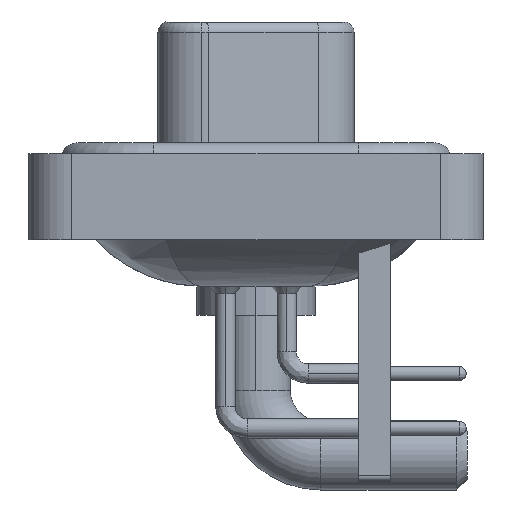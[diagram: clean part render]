
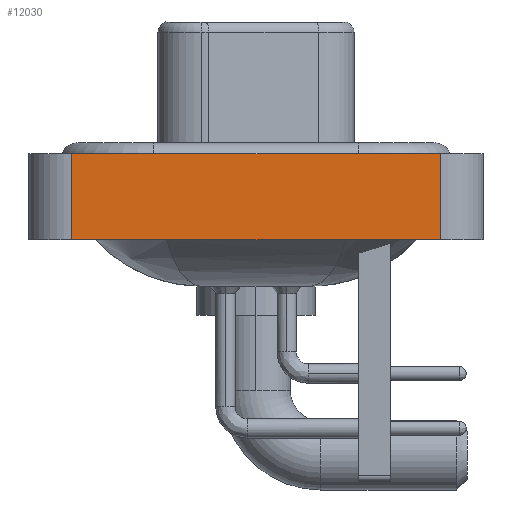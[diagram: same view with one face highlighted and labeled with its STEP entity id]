
A CAD part, left-side view. The second image highlights one B-rep face of the part: STEP entity #12030.
In plain terms, the highlighted planar face has unit normal (-1, 0, 0).
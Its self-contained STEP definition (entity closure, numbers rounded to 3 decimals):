
#790 = DIRECTION ( 'NONE',  ( 0., 0., 1. ) ) ;
#1094 = FACE_OUTER_BOUND ( 'NONE', #12705, .T. ) ;
#1133 = CARTESIAN_POINT ( 'NONE',  ( -7.3, 8.55, -3.6 ) ) ;
#2827 = CARTESIAN_POINT ( 'NONE',  ( -7.3, -8.55, 0.4 ) ) ;
#2832 = CARTESIAN_POINT ( 'NONE',  ( -7.3, -8.55, -3.6 ) ) ;
#3358 = EDGE_CURVE ( 'NONE', #23536, #13265, #13192, .T. ) ;
#3479 = CARTESIAN_POINT ( 'NONE',  ( -7.3, -8.55, -3.6 ) ) ;
#3744 = VERTEX_POINT ( 'NONE', #9728 ) ;
#3817 = VECTOR ( 'NONE', #11055, 1000. ) ;
#4490 = DIRECTION ( 'NONE',  ( 0., -1., 0. ) ) ;
#4636 = VECTOR ( 'NONE', #790, 1000. ) ;
#6869 = PLANE ( 'NONE',  #13501 ) ;
#7270 = DIRECTION ( 'NONE',  ( 0., 0., 1. ) ) ;
#9379 = EDGE_CURVE ( 'NONE', #3744, #13265, #21364, .T. ) ;
#9728 = CARTESIAN_POINT ( 'NONE',  ( -7.3, 8.55, 0.4 ) ) ;
#10566 = VECTOR ( 'NONE', #23372, 1000. ) ;
#11055 = DIRECTION ( 'NONE',  ( 0., -1., 0. ) ) ;
#11863 = VECTOR ( 'NONE', #4490, 1000. ) ;
#12030 = ADVANCED_FACE ( 'NONE', ( #1094 ), #6869, .T. ) ;
#12705 = EDGE_LOOP ( 'NONE', ( #26020, #24144, #25763, #20966 ) ) ;
#13192 = LINE ( 'NONE', #16997, #4636 ) ;
#13265 = VERTEX_POINT ( 'NONE', #19517 ) ;
#13479 = VERTEX_POINT ( 'NONE', #1133 ) ;
#13501 = AXIS2_PLACEMENT_3D ( 'NONE', #2832, #25857, #7270 ) ;
#14255 = EDGE_CURVE ( 'NONE', #13479, #3744, #19141, .T. ) ;
#16997 = CARTESIAN_POINT ( 'NONE',  ( -7.3, -8.55, -3.6 ) ) ;
#18861 = LINE ( 'NONE', #25237, #11863 ) ;
#19001 = EDGE_CURVE ( 'NONE', #13479, #23536, #18861, .T. ) ;
#19141 = LINE ( 'NONE', #25391, #10566 ) ;
#19517 = CARTESIAN_POINT ( 'NONE',  ( -7.3, -8.55, 0.4 ) ) ;
#20966 = ORIENTED_EDGE ( 'NONE', *, *, #19001, .T. ) ;
#21364 = LINE ( 'NONE', #2827, #3817 ) ;
#23372 = DIRECTION ( 'NONE',  ( 0., 0., 1. ) ) ;
#23536 = VERTEX_POINT ( 'NONE', #3479 ) ;
#24144 = ORIENTED_EDGE ( 'NONE', *, *, #9379, .F. ) ;
#25237 = CARTESIAN_POINT ( 'NONE',  ( -7.3, -8.55, -3.6 ) ) ;
#25391 = CARTESIAN_POINT ( 'NONE',  ( -7.3, 8.55, -3.6 ) ) ;
#25763 = ORIENTED_EDGE ( 'NONE', *, *, #14255, .F. ) ;
#25857 = DIRECTION ( 'NONE',  ( -1., 0., 0. ) ) ;
#26020 = ORIENTED_EDGE ( 'NONE', *, *, #3358, .T. ) ;
